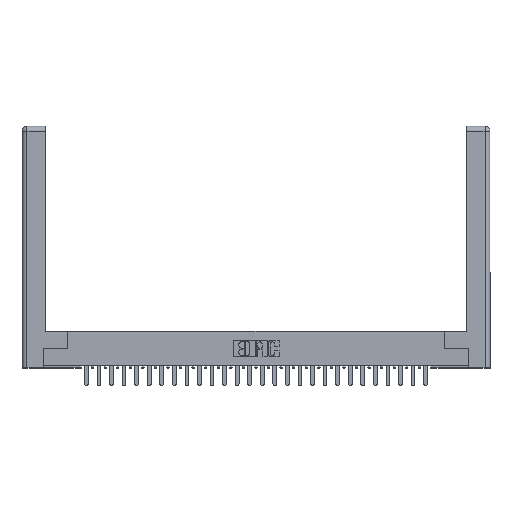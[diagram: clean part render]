
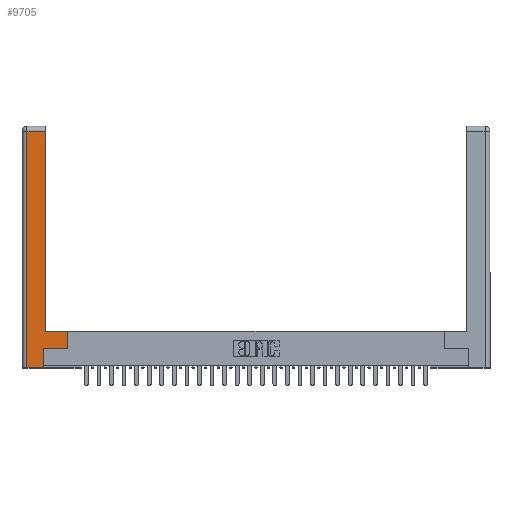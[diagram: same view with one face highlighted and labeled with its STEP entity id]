
A CAD part, top view. The second image highlights one B-rep face of the part: STEP entity #9705.
In plain terms, the highlighted planar face has unit normal (0, 0, 1).
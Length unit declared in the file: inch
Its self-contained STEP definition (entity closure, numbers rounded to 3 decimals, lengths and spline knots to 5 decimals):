
#1026 = CARTESIAN_POINT ( 'NONE',  ( 0.265, 0.245, 0. ) ) ;
#2469 = LINE ( 'NONE', #3118, #7343 ) ;
#3118 = CARTESIAN_POINT ( 'NONE',  ( 0.265, 0., 0. ) ) ;
#3214 = DIRECTION ( 'NONE',  ( -1., 0., 0. ) ) ;
#3500 = VERTEX_POINT ( 'NONE', #19798 ) ;
#3512 = ORIENTED_EDGE ( 'NONE', *, *, #25595, .T. ) ;
#5244 = VECTOR ( 'NONE', #28273, 39.37008 ) ;
#5856 = CARTESIAN_POINT ( 'NONE',  ( 0., 0., 0. ) ) ;
#6304 = VERTEX_POINT ( 'NONE', #18235 ) ;
#6904 = VERTEX_POINT ( 'NONE', #24132 ) ;
#7343 = VECTOR ( 'NONE', #21932, 39.37008 ) ;
#8246 = DIRECTION ( 'NONE',  ( -1., 0., 0. ) ) ;
#8335 = ORIENTED_EDGE ( 'NONE', *, *, #15586, .T. ) ;
#8437 = LINE ( 'NONE', #21184, #26401 ) ;
#9203 = DIRECTION ( 'NONE',  ( 1., 0., 0. ) ) ;
#9337 = LINE ( 'NONE', #19575, #21754 ) ;
#9524 = CARTESIAN_POINT ( 'NONE',  ( 0.565, 0.45, 0. ) ) ;
#9694 = VERTEX_POINT ( 'NONE', #1026 ) ;
#9705 = ADVANCED_FACE ( 'NONE', ( #24709 ), #29229, .F. ) ;
#9937 = EDGE_CURVE ( 'NONE', #6304, #3500, #18829, .T. ) ;
#10001 = CARTESIAN_POINT ( 'NONE',  ( 0.565, 0.245, 0. ) ) ;
#11292 = ORIENTED_EDGE ( 'NONE', *, *, #26729, .T. ) ;
#11414 = DIRECTION ( 'NONE',  ( 0., -1., 0. ) ) ;
#11528 = LINE ( 'NONE', #9524, #5244 ) ;
#11542 = VECTOR ( 'NONE', #9203, 39.37008 ) ;
#12293 = ORIENTED_EDGE ( 'NONE', *, *, #9937, .T. ) ;
#12719 = CARTESIAN_POINT ( 'NONE',  ( 0.295, 2.94, 0. ) ) ;
#14004 = ORIENTED_EDGE ( 'NONE', *, *, #18734, .T. ) ;
#14353 = LINE ( 'NONE', #15287, #19833 ) ;
#14949 = CARTESIAN_POINT ( 'NONE',  ( 0.295, 0.45, 0. ) ) ;
#15287 = CARTESIAN_POINT ( 'NONE',  ( 0.265, 0.245, 0. ) ) ;
#15341 = ORIENTED_EDGE ( 'NONE', *, *, #29879, .T. ) ;
#15586 = EDGE_CURVE ( 'NONE', #3500, #30268, #2469, .T. ) ;
#17644 = DIRECTION ( 'NONE',  ( 0., 1., 0. ) ) ;
#18235 = CARTESIAN_POINT ( 'NONE',  ( 0.0615, 2.94, 0. ) ) ;
#18499 = CARTESIAN_POINT ( 'NONE',  ( 0.565, 0.245, 0. ) ) ;
#18734 = EDGE_CURVE ( 'NONE', #26537, #19066, #11528, .T. ) ;
#18829 = LINE ( 'NONE', #25426, #29840 ) ;
#18951 = DIRECTION ( 'NONE',  ( 0., 1., 0. ) ) ;
#19066 = VERTEX_POINT ( 'NONE', #22477 ) ;
#19389 = DIRECTION ( 'NONE',  ( -1., 0., 0. ) ) ;
#19575 = CARTESIAN_POINT ( 'NONE',  ( 0.0615, 2.94, 0. ) ) ;
#19798 = CARTESIAN_POINT ( 'NONE',  ( 0.0615, 0., 0. ) ) ;
#19833 = VECTOR ( 'NONE', #17644, 39.37008 ) ;
#20272 = VECTOR ( 'NONE', #3214, 39.37008 ) ;
#20928 = EDGE_CURVE ( 'NONE', #6904, #29055, #8437, .T. ) ;
#21012 = LINE ( 'NONE', #14949, #20272 ) ;
#21107 = EDGE_LOOP ( 'NONE', ( #25097, #3512, #12293, #8335, #11292, #15341, #14004, #26703 ) ) ;
#21184 = CARTESIAN_POINT ( 'NONE',  ( 0.295, 3., 0. ) ) ;
#21754 = VECTOR ( 'NONE', #19389, 39.37008 ) ;
#21932 = DIRECTION ( 'NONE',  ( 1., 0., 0. ) ) ;
#22250 = DIRECTION ( 'NONE',  ( 0., 0., -1. ) ) ;
#22477 = CARTESIAN_POINT ( 'NONE',  ( 0.565, 0.45, 0. ) ) ;
#24132 = CARTESIAN_POINT ( 'NONE',  ( 0.295, 0.45, 0. ) ) ;
#24709 = FACE_OUTER_BOUND ( 'NONE', #21107, .T. ) ;
#25097 = ORIENTED_EDGE ( 'NONE', *, *, #20928, .T. ) ;
#25426 = CARTESIAN_POINT ( 'NONE',  ( 0.0615, 0., 0. ) ) ;
#25595 = EDGE_CURVE ( 'NONE', #29055, #6304, #9337, .T. ) ;
#25621 = EDGE_CURVE ( 'NONE', #19066, #6904, #21012, .T. ) ;
#26401 = VECTOR ( 'NONE', #18951, 39.37008 ) ;
#26537 = VERTEX_POINT ( 'NONE', #10001 ) ;
#26703 = ORIENTED_EDGE ( 'NONE', *, *, #25621, .T. ) ;
#26729 = EDGE_CURVE ( 'NONE', #30268, #9694, #14353, .T. ) ;
#27901 = AXIS2_PLACEMENT_3D ( 'NONE', #5856, #22250, #8246 ) ;
#28273 = DIRECTION ( 'NONE',  ( 0., 1., 0. ) ) ;
#29055 = VERTEX_POINT ( 'NONE', #12719 ) ;
#29229 = PLANE ( 'NONE',  #27901 ) ;
#29336 = CARTESIAN_POINT ( 'NONE',  ( 0.265, 0., 0. ) ) ;
#29487 = LINE ( 'NONE', #18499, #11542 ) ;
#29840 = VECTOR ( 'NONE', #11414, 39.37008 ) ;
#29879 = EDGE_CURVE ( 'NONE', #9694, #26537, #29487, .T. ) ;
#30268 = VERTEX_POINT ( 'NONE', #29336 ) ;
